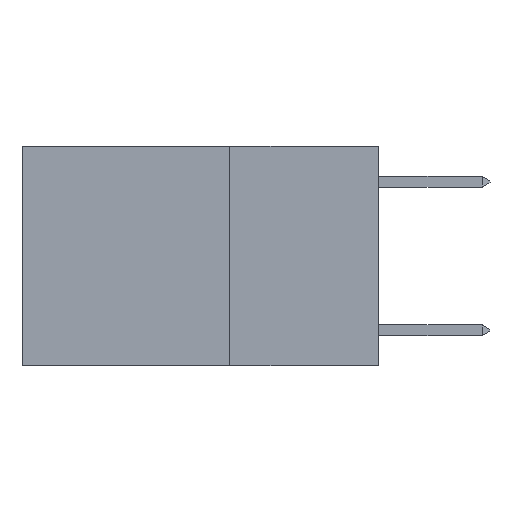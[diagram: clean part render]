
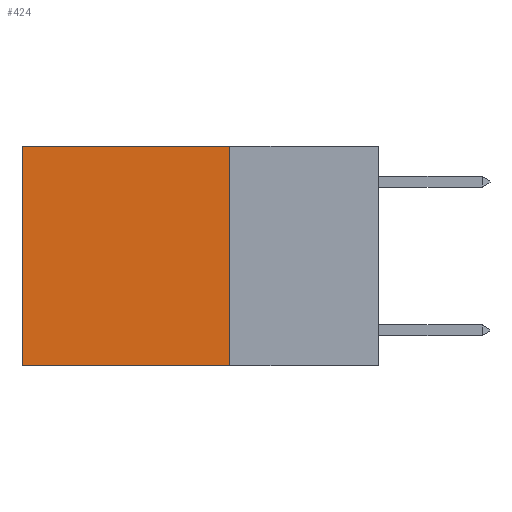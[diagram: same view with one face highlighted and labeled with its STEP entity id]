
A CAD part, left-side view. The second image highlights one B-rep face of the part: STEP entity #424.
In plain terms, the highlighted planar face has unit normal (-1, 0, 0).
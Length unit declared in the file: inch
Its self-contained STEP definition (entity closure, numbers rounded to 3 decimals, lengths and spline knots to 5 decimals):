
#90 = VERTEX_POINT ( 'NONE', #2128 ) ;
#91 = ORIENTED_EDGE ( 'NONE', *, *, #5733, .F. ) ;
#424 = ADVANCED_FACE ( 'NONE', ( #8646 ), #7863, .F. ) ;
#437 = LINE ( 'NONE', #2672, #2770 ) ;
#1584 = VERTEX_POINT ( 'NONE', #5833 ) ;
#1683 = VECTOR ( 'NONE', #5254, 39.37008 ) ;
#1717 = VECTOR ( 'NONE', #4264, 39.37008 ) ;
#1819 = CARTESIAN_POINT ( 'NONE',  ( 0.2625, 0.25, 0. ) ) ;
#1868 = EDGE_LOOP ( 'NONE', ( #2601, #91, #3058, #3970 ) ) ;
#1958 = DIRECTION ( 'NONE',  ( 0., 0., -1. ) ) ;
#2128 = CARTESIAN_POINT ( 'NONE',  ( 0.2625, 0.25, -0.37 ) ) ;
#2328 = EDGE_CURVE ( 'NONE', #8600, #90, #437, .T. ) ;
#2601 = ORIENTED_EDGE ( 'NONE', *, *, #9438, .T. ) ;
#2672 = CARTESIAN_POINT ( 'NONE',  ( 0.2625, 0.25, 0. ) ) ;
#2770 = VECTOR ( 'NONE', #4158, 39.37008 ) ;
#3026 = EDGE_CURVE ( 'NONE', #8600, #1584, #8749, .T. ) ;
#3058 = ORIENTED_EDGE ( 'NONE', *, *, #2328, .F. ) ;
#3089 = LINE ( 'NONE', #5307, #1683 ) ;
#3443 = AXIS2_PLACEMENT_3D ( 'NONE', #1819, #9338, #1958 ) ;
#3526 = LINE ( 'NONE', #4845, #1717 ) ;
#3619 = CARTESIAN_POINT ( 'NONE',  ( 0.2625, 0.25, 0. ) ) ;
#3970 = ORIENTED_EDGE ( 'NONE', *, *, #3026, .T. ) ;
#3995 = CARTESIAN_POINT ( 'NONE',  ( 0.2625, 0.6, -0.37 ) ) ;
#4008 = VECTOR ( 'NONE', #7332, 39.37008 ) ;
#4158 = DIRECTION ( 'NONE',  ( 0., 0., -1. ) ) ;
#4264 = DIRECTION ( 'NONE',  ( 0., 1., 0. ) ) ;
#4845 = CARTESIAN_POINT ( 'NONE',  ( 0.2625, 0.25, -0.37 ) ) ;
#5254 = DIRECTION ( 'NONE',  ( 0., 0., -1. ) ) ;
#5307 = CARTESIAN_POINT ( 'NONE',  ( 0.2625, 0.6, 0. ) ) ;
#5733 = EDGE_CURVE ( 'NONE', #90, #9571, #3526, .T. ) ;
#5833 = CARTESIAN_POINT ( 'NONE',  ( 0.2625, 0.6, 0. ) ) ;
#6988 = CARTESIAN_POINT ( 'NONE',  ( 0.2625, 0.25, 0. ) ) ;
#7332 = DIRECTION ( 'NONE',  ( 0., 1., 0. ) ) ;
#7863 = PLANE ( 'NONE',  #3443 ) ;
#8600 = VERTEX_POINT ( 'NONE', #6988 ) ;
#8646 = FACE_OUTER_BOUND ( 'NONE', #1868, .T. ) ;
#8749 = LINE ( 'NONE', #3619, #4008 ) ;
#9338 = DIRECTION ( 'NONE',  ( 1., 0., 0. ) ) ;
#9438 = EDGE_CURVE ( 'NONE', #1584, #9571, #3089, .T. ) ;
#9571 = VERTEX_POINT ( 'NONE', #3995 ) ;
